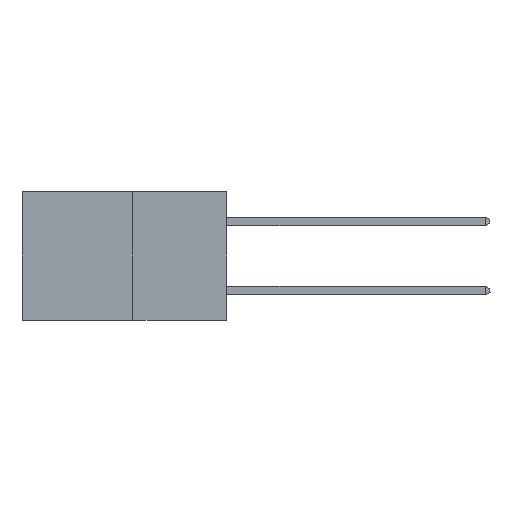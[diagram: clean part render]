
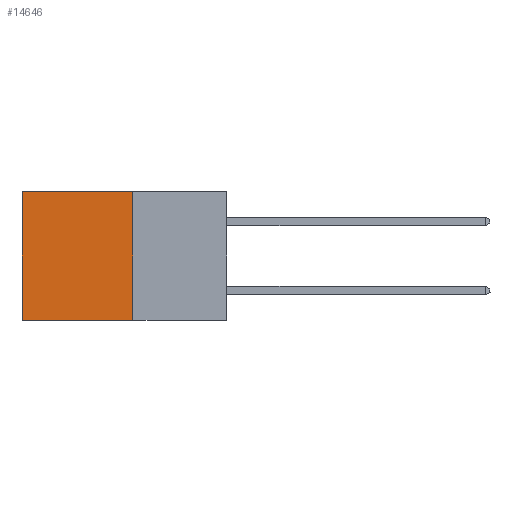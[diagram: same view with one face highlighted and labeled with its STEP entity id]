
A CAD part, left-side view. The second image highlights one B-rep face of the part: STEP entity #14646.
In plain terms, the highlighted planar face has unit normal (-1, 0, 0).
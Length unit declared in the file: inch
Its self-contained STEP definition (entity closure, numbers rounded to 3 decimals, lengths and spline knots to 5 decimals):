
#908 = ORIENTED_EDGE ( 'NONE', *, *, #9453, .F. ) ;
#1480 = VECTOR ( 'NONE', #12297, 39.37008 ) ;
#2371 = ORIENTED_EDGE ( 'NONE', *, *, #8343, .T. ) ;
#2429 = VECTOR ( 'NONE', #5501, 39.37008 ) ;
#2970 = AXIS2_PLACEMENT_3D ( 'NONE', #13951, #12761, #5286 ) ;
#3139 = VERTEX_POINT ( 'NONE', #4461 ) ;
#3796 = EDGE_CURVE ( 'NONE', #3139, #6189, #4194, .T. ) ;
#4068 = PLANE ( 'NONE',  #2970 ) ;
#4194 = LINE ( 'NONE', #16010, #12962 ) ;
#4461 = CARTESIAN_POINT ( 'NONE',  ( 0.277, 0.27, 0. ) ) ;
#4617 = EDGE_LOOP ( 'NONE', ( #2371, #12077, #908, #5889 ) ) ;
#5286 = DIRECTION ( 'NONE',  ( 0., 0., -1. ) ) ;
#5501 = DIRECTION ( 'NONE',  ( 0., 0., -1. ) ) ;
#5889 = ORIENTED_EDGE ( 'NONE', *, *, #3796, .T. ) ;
#6189 = VERTEX_POINT ( 'NONE', #10594 ) ;
#7139 = EDGE_CURVE ( 'NONE', #7907, #10441, #10890, .T. ) ;
#7574 = VECTOR ( 'NONE', #13505, 39.37008 ) ;
#7907 = VERTEX_POINT ( 'NONE', #9157 ) ;
#8343 = EDGE_CURVE ( 'NONE', #6189, #10441, #11808, .T. ) ;
#9157 = CARTESIAN_POINT ( 'NONE',  ( 0.277, 0.27, -0.37 ) ) ;
#9435 = DIRECTION ( 'NONE',  ( 0., 1., 0. ) ) ;
#9453 = EDGE_CURVE ( 'NONE', #3139, #7907, #15997, .T. ) ;
#10441 = VERTEX_POINT ( 'NONE', #12570 ) ;
#10594 = CARTESIAN_POINT ( 'NONE',  ( 0.277, 0.59, 0. ) ) ;
#10890 = LINE ( 'NONE', #10996, #7574 ) ;
#10996 = CARTESIAN_POINT ( 'NONE',  ( 0.277, 0.27, -0.37 ) ) ;
#11033 = CARTESIAN_POINT ( 'NONE',  ( 0.277, 0.59, -0.37 ) ) ;
#11743 = CARTESIAN_POINT ( 'NONE',  ( 0.277, 0.27, -0.37 ) ) ;
#11808 = LINE ( 'NONE', #11033, #1480 ) ;
#12077 = ORIENTED_EDGE ( 'NONE', *, *, #7139, .F. ) ;
#12297 = DIRECTION ( 'NONE',  ( 0., 0., -1. ) ) ;
#12570 = CARTESIAN_POINT ( 'NONE',  ( 0.277, 0.59, -0.37 ) ) ;
#12761 = DIRECTION ( 'NONE',  ( 1., 0., 0. ) ) ;
#12962 = VECTOR ( 'NONE', #9435, 39.37008 ) ;
#13087 = FACE_OUTER_BOUND ( 'NONE', #4617, .T. ) ;
#13505 = DIRECTION ( 'NONE',  ( 0., 1., 0. ) ) ;
#13951 = CARTESIAN_POINT ( 'NONE',  ( 0.277, 0.27, -0.37 ) ) ;
#14646 = ADVANCED_FACE ( 'NONE', ( #13087 ), #4068, .F. ) ;
#15997 = LINE ( 'NONE', #11743, #2429 ) ;
#16010 = CARTESIAN_POINT ( 'NONE',  ( 0.277, 0.27, 0. ) ) ;
